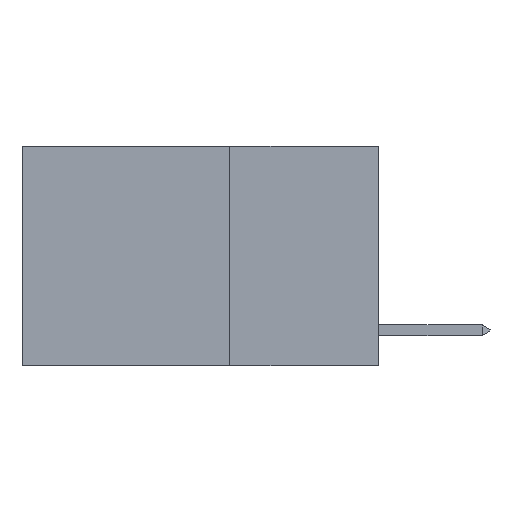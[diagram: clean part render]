
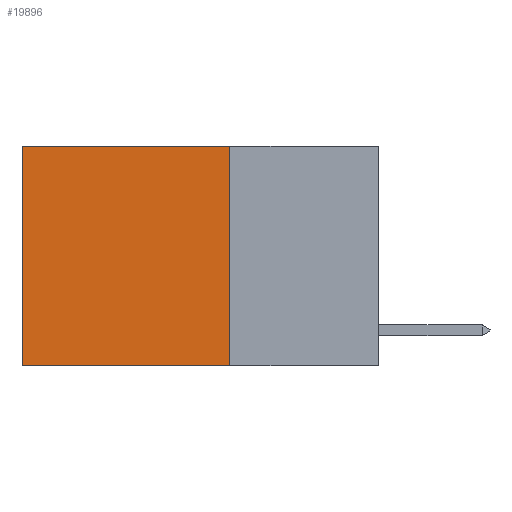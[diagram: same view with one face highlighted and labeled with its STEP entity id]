
A CAD part, left-side view. The second image highlights one B-rep face of the part: STEP entity #19896.
In plain terms, the highlighted planar face has unit normal (-1, 0, 0).
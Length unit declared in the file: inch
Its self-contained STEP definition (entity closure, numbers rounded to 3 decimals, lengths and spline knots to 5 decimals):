
#2553 = CARTESIAN_POINT ( 'NONE',  ( 0.2625, 0.6, -0.37 ) ) ;
#4345 = CARTESIAN_POINT ( 'NONE',  ( 0.2625, 0.6, 0. ) ) ;
#4432 = EDGE_LOOP ( 'NONE', ( #23379, #13999, #21640, #10068 ) ) ;
#4745 = CARTESIAN_POINT ( 'NONE',  ( 0.2625, 0.6, 0. ) ) ;
#4760 = CARTESIAN_POINT ( 'NONE',  ( 0.2625, 0.25, 0. ) ) ;
#6641 = EDGE_CURVE ( 'NONE', #7336, #10889, #24147, .T. ) ;
#7336 = VERTEX_POINT ( 'NONE', #4345 ) ;
#7656 = DIRECTION ( 'NONE',  ( 0., 0., -1. ) ) ;
#7713 = VECTOR ( 'NONE', #7656, 39.37008 ) ;
#7889 = AXIS2_PLACEMENT_3D ( 'NONE', #13107, #21927, #15143 ) ;
#8164 = FACE_OUTER_BOUND ( 'NONE', #4432, .T. ) ;
#10068 = ORIENTED_EDGE ( 'NONE', *, *, #16671, .T. ) ;
#10171 = VECTOR ( 'NONE', #11562, 39.37008 ) ;
#10889 = VERTEX_POINT ( 'NONE', #2553 ) ;
#11562 = DIRECTION ( 'NONE',  ( 0., 1., 0. ) ) ;
#11609 = EDGE_CURVE ( 'NONE', #25979, #23848, #22869, .T. ) ;
#12436 = DIRECTION ( 'NONE',  ( 0., 1., 0. ) ) ;
#13107 = CARTESIAN_POINT ( 'NONE',  ( 0.2625, 0.25, 0. ) ) ;
#13579 = EDGE_CURVE ( 'NONE', #23848, #10889, #21522, .T. ) ;
#13999 = ORIENTED_EDGE ( 'NONE', *, *, #13579, .F. ) ;
#15143 = DIRECTION ( 'NONE',  ( 0., 0., -1. ) ) ;
#15708 = VECTOR ( 'NONE', #15897, 39.37008 ) ;
#15897 = DIRECTION ( 'NONE',  ( 0., 0., -1. ) ) ;
#16671 = EDGE_CURVE ( 'NONE', #25979, #7336, #22404, .T. ) ;
#16825 = CARTESIAN_POINT ( 'NONE',  ( 0.2625, 0.25, 0. ) ) ;
#18822 = CARTESIAN_POINT ( 'NONE',  ( 0.2625, 0.25, 0. ) ) ;
#19297 = VECTOR ( 'NONE', #12436, 39.37008 ) ;
#19896 = ADVANCED_FACE ( 'NONE', ( #8164 ), #24103, .F. ) ;
#21356 = CARTESIAN_POINT ( 'NONE',  ( 0.2625, 0.25, -0.37 ) ) ;
#21522 = LINE ( 'NONE', #23262, #19297 ) ;
#21640 = ORIENTED_EDGE ( 'NONE', *, *, #11609, .F. ) ;
#21927 = DIRECTION ( 'NONE',  ( 1., 0., 0. ) ) ;
#22404 = LINE ( 'NONE', #4760, #10171 ) ;
#22869 = LINE ( 'NONE', #18822, #7713 ) ;
#23262 = CARTESIAN_POINT ( 'NONE',  ( 0.2625, 0.25, -0.37 ) ) ;
#23379 = ORIENTED_EDGE ( 'NONE', *, *, #6641, .T. ) ;
#23848 = VERTEX_POINT ( 'NONE', #21356 ) ;
#24103 = PLANE ( 'NONE',  #7889 ) ;
#24147 = LINE ( 'NONE', #4745, #15708 ) ;
#25979 = VERTEX_POINT ( 'NONE', #16825 ) ;
